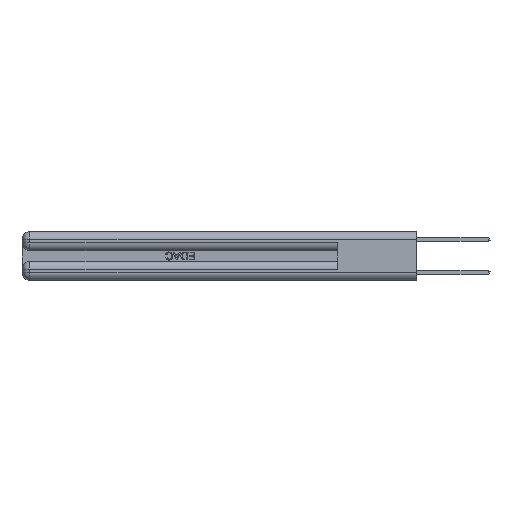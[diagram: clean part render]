
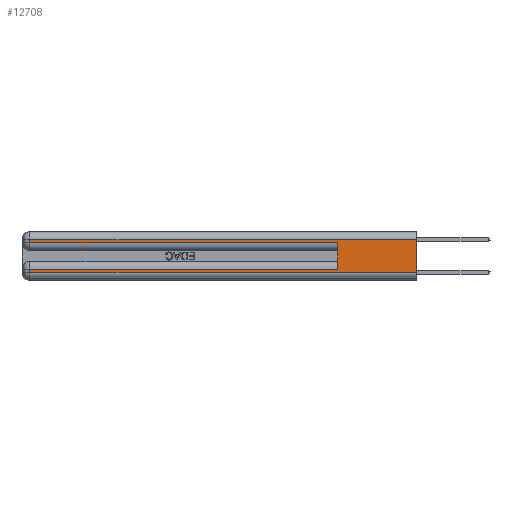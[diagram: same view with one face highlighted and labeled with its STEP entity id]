
A CAD part, left-side view. The second image highlights one B-rep face of the part: STEP entity #12708.
In plain terms, the highlighted planar face has unit normal (-1, 0, 0).
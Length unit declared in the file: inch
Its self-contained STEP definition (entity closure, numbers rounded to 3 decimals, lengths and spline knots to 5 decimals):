
#9 = EDGE_CURVE ( 'NONE', #23859, #12756, #24096, .T. ) ;
#451 = CARTESIAN_POINT ( 'NONE',  ( 0., 0., 0.085 ) ) ;
#1084 = EDGE_CURVE ( 'NONE', #23588, #15220, #6070, .T. ) ;
#1724 = DIRECTION ( 'NONE',  ( 0., 0., -1. ) ) ;
#2731 = CARTESIAN_POINT ( 'NONE',  ( 0., 0.6, 0.285 ) ) ;
#3709 = ORIENTED_EDGE ( 'NONE', *, *, #17947, .T. ) ;
#5268 = ORIENTED_EDGE ( 'NONE', *, *, #9792, .T. ) ;
#5623 = CARTESIAN_POINT ( 'NONE',  ( 0., 0., 0.06 ) ) ;
#5678 = CARTESIAN_POINT ( 'NONE',  ( 0., 0., 0.37 ) ) ;
#5835 = DIRECTION ( 'NONE',  ( 0., 0., -1. ) ) ;
#5847 = VECTOR ( 'NONE', #24381, 39.37008 ) ;
#6070 = LINE ( 'NONE', #6410, #34090 ) ;
#6377 = VECTOR ( 'NONE', #15652, 39.37008 ) ;
#6404 = ORIENTED_EDGE ( 'NONE', *, *, #33248, .F. ) ;
#6410 = CARTESIAN_POINT ( 'NONE',  ( 0., 0., 0.31 ) ) ;
#6978 = PLANE ( 'NONE',  #28620 ) ;
#7315 = CARTESIAN_POINT ( 'NONE',  ( 0., 2.94, 0.285 ) ) ;
#7875 = VECTOR ( 'NONE', #19103, 39.37008 ) ;
#8118 = EDGE_CURVE ( 'NONE', #26736, #12026, #29087, .T. ) ;
#8523 = LINE ( 'NONE', #24213, #18559 ) ;
#9270 = VERTEX_POINT ( 'NONE', #2731 ) ;
#9651 = ORIENTED_EDGE ( 'NONE', *, *, #9, .T. ) ;
#9792 = EDGE_CURVE ( 'NONE', #26061, #9270, #8523, .T. ) ;
#9825 = CARTESIAN_POINT ( 'NONE',  ( 0., 2.94, 0.06 ) ) ;
#11129 = DIRECTION ( 'NONE',  ( 0., -1., 0. ) ) ;
#12026 = VERTEX_POINT ( 'NONE', #28156 ) ;
#12708 = ADVANCED_FACE ( 'NONE', ( #22688 ), #6978, .F. ) ;
#12756 = VERTEX_POINT ( 'NONE', #24816 ) ;
#13877 = LINE ( 'NONE', #22296, #5847 ) ;
#14696 = DIRECTION ( 'NONE',  ( 0., 1., 0. ) ) ;
#14970 = VECTOR ( 'NONE', #5835, 39.37008 ) ;
#15220 = VERTEX_POINT ( 'NONE', #27609 ) ;
#15652 = DIRECTION ( 'NONE',  ( 0., -1., 0. ) ) ;
#16827 = EDGE_CURVE ( 'NONE', #23588, #12026, #32084, .T. ) ;
#17826 = EDGE_CURVE ( 'NONE', #12756, #26736, #25031, .T. ) ;
#17947 = EDGE_CURVE ( 'NONE', #15220, #26061, #33987, .T. ) ;
#18559 = VECTOR ( 'NONE', #11129, 39.37008 ) ;
#19103 = DIRECTION ( 'NONE',  ( 0., 1., 0. ) ) ;
#19132 = CARTESIAN_POINT ( 'NONE',  ( 0., 0., 0.37 ) ) ;
#19864 = ORIENTED_EDGE ( 'NONE', *, *, #16827, .F. ) ;
#20582 = CARTESIAN_POINT ( 'NONE',  ( 0., 0., 0.31 ) ) ;
#22057 = DIRECTION ( 'NONE',  ( 0., 0., -1. ) ) ;
#22262 = EDGE_LOOP ( 'NONE', ( #19864, #30383, #3709, #5268, #6404, #9651, #24898, #23176 ) ) ;
#22296 = CARTESIAN_POINT ( 'NONE',  ( 0., 0.6, 0.145 ) ) ;
#22688 = FACE_OUTER_BOUND ( 'NONE', #22262, .T. ) ;
#23112 = CARTESIAN_POINT ( 'NONE',  ( 0., 2.94, 0.37 ) ) ;
#23176 = ORIENTED_EDGE ( 'NONE', *, *, #8118, .T. ) ;
#23588 = VERTEX_POINT ( 'NONE', #20582 ) ;
#23859 = VERTEX_POINT ( 'NONE', #29702 ) ;
#24096 = LINE ( 'NONE', #451, #7875 ) ;
#24213 = CARTESIAN_POINT ( 'NONE',  ( 0., 0., 0.285 ) ) ;
#24381 = DIRECTION ( 'NONE',  ( 0., 0., 1. ) ) ;
#24816 = CARTESIAN_POINT ( 'NONE',  ( 0., 2.94, 0.085 ) ) ;
#24898 = ORIENTED_EDGE ( 'NONE', *, *, #17826, .T. ) ;
#25031 = LINE ( 'NONE', #26998, #29880 ) ;
#26061 = VERTEX_POINT ( 'NONE', #7315 ) ;
#26736 = VERTEX_POINT ( 'NONE', #9825 ) ;
#26998 = CARTESIAN_POINT ( 'NONE',  ( 0., 2.94, 0.37 ) ) ;
#27609 = CARTESIAN_POINT ( 'NONE',  ( 0., 2.94, 0.31 ) ) ;
#28156 = CARTESIAN_POINT ( 'NONE',  ( 0., 0., 0.06 ) ) ;
#28301 = DIRECTION ( 'NONE',  ( 0., 0., -1. ) ) ;
#28620 = AXIS2_PLACEMENT_3D ( 'NONE', #19132, #29641, #22057 ) ;
#29087 = LINE ( 'NONE', #5623, #6377 ) ;
#29338 = VECTOR ( 'NONE', #28301, 39.37008 ) ;
#29641 = DIRECTION ( 'NONE',  ( 1., 0., 0. ) ) ;
#29702 = CARTESIAN_POINT ( 'NONE',  ( 0., 0.6, 0.085 ) ) ;
#29880 = VECTOR ( 'NONE', #1724, 39.37008 ) ;
#30383 = ORIENTED_EDGE ( 'NONE', *, *, #1084, .T. ) ;
#32084 = LINE ( 'NONE', #5678, #14970 ) ;
#33248 = EDGE_CURVE ( 'NONE', #23859, #9270, #13877, .T. ) ;
#33987 = LINE ( 'NONE', #23112, #29338 ) ;
#34090 = VECTOR ( 'NONE', #14696, 39.37008 ) ;
